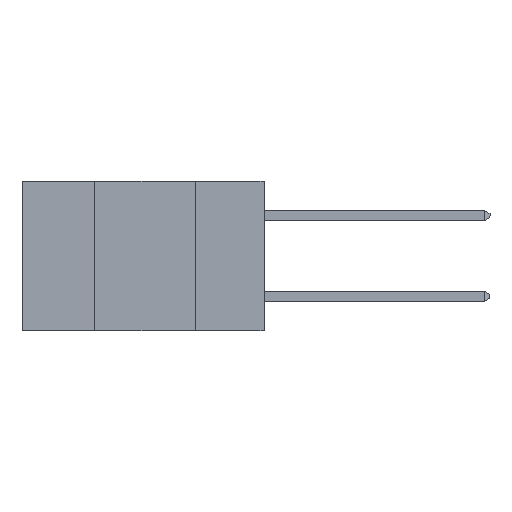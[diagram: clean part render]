
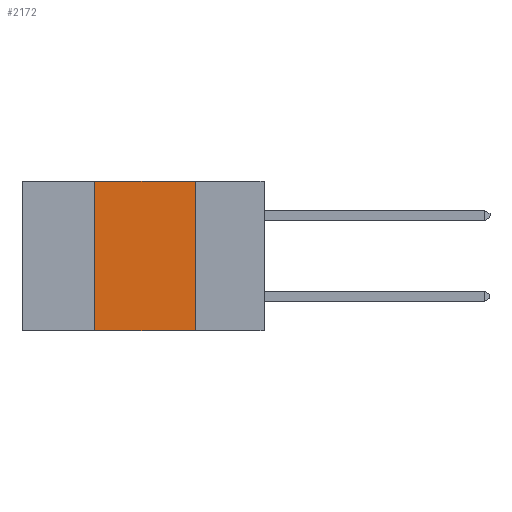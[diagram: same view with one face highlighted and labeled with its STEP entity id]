
A CAD part, left-side view. The second image highlights one B-rep face of the part: STEP entity #2172.
In plain terms, the highlighted planar face has unit normal (-1, 0, 0).
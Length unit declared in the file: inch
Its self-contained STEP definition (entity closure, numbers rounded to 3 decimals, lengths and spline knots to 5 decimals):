
#793 = CARTESIAN_POINT ( 'NONE',  ( 0., 0.6, -0.37 ) ) ;
#880 = PLANE ( 'NONE',  #3057 ) ;
#895 = DIRECTION ( 'NONE',  ( 0., 0., -1. ) ) ;
#946 = EDGE_LOOP ( 'NONE', ( #2364, #2455, #2478, #2598 ) ) ;
#1075 = VECTOR ( 'NONE', #2831, 39.37008 ) ;
#1314 = CARTESIAN_POINT ( 'NONE',  ( 0., 0.6, 0. ) ) ;
#1571 = CARTESIAN_POINT ( 'NONE',  ( 0., 0.17, 0. ) ) ;
#2172 = ADVANCED_FACE ( 'NONE', ( #6714 ), #880, .F. ) ;
#2364 = ORIENTED_EDGE ( 'NONE', *, *, #9897, .F. ) ;
#2374 = DIRECTION ( 'NONE',  ( 1., 0., 0. ) ) ;
#2415 = CARTESIAN_POINT ( 'NONE',  ( 0., 0.17, -0.37 ) ) ;
#2455 = ORIENTED_EDGE ( 'NONE', *, *, #3105, .F. ) ;
#2478 = ORIENTED_EDGE ( 'NONE', *, *, #7893, .F. ) ;
#2598 = ORIENTED_EDGE ( 'NONE', *, *, #5875, .T. ) ;
#2701 = CARTESIAN_POINT ( 'NONE',  ( 0., 0.42, 0. ) ) ;
#2831 = DIRECTION ( 'NONE',  ( 0., 0., 1. ) ) ;
#3057 = AXIS2_PLACEMENT_3D ( 'NONE', #12402, #2374, #895 ) ;
#3105 = EDGE_CURVE ( 'NONE', #6864, #6482, #9339, .T. ) ;
#3650 = LINE ( 'NONE', #6210, #10724 ) ;
#4981 = VERTEX_POINT ( 'NONE', #12833 ) ;
#5875 = EDGE_CURVE ( 'NONE', #4981, #6527, #7075, .T. ) ;
#6210 = CARTESIAN_POINT ( 'NONE',  ( 0., 0.17, 0. ) ) ;
#6482 = VERTEX_POINT ( 'NONE', #1571 ) ;
#6527 = VERTEX_POINT ( 'NONE', #2415 ) ;
#6687 = VECTOR ( 'NONE', #11752, 39.37008 ) ;
#6714 = FACE_OUTER_BOUND ( 'NONE', #946, .T. ) ;
#6864 = VERTEX_POINT ( 'NONE', #10761 ) ;
#7075 = LINE ( 'NONE', #793, #9729 ) ;
#7893 = EDGE_CURVE ( 'NONE', #4981, #6864, #11892, .T. ) ;
#9339 = LINE ( 'NONE', #1314, #6687 ) ;
#9729 = VECTOR ( 'NONE', #9818, 39.37008 ) ;
#9818 = DIRECTION ( 'NONE',  ( 0., -1., 0. ) ) ;
#9897 = EDGE_CURVE ( 'NONE', #6482, #6527, #3650, .T. ) ;
#10724 = VECTOR ( 'NONE', #11258, 39.37008 ) ;
#10761 = CARTESIAN_POINT ( 'NONE',  ( 0., 0.42, 0. ) ) ;
#11258 = DIRECTION ( 'NONE',  ( 0., 0., -1. ) ) ;
#11752 = DIRECTION ( 'NONE',  ( 0., -1., 0. ) ) ;
#11892 = LINE ( 'NONE', #2701, #1075 ) ;
#12402 = CARTESIAN_POINT ( 'NONE',  ( 0., 0.6, 0. ) ) ;
#12833 = CARTESIAN_POINT ( 'NONE',  ( 0., 0.42, -0.37 ) ) ;
